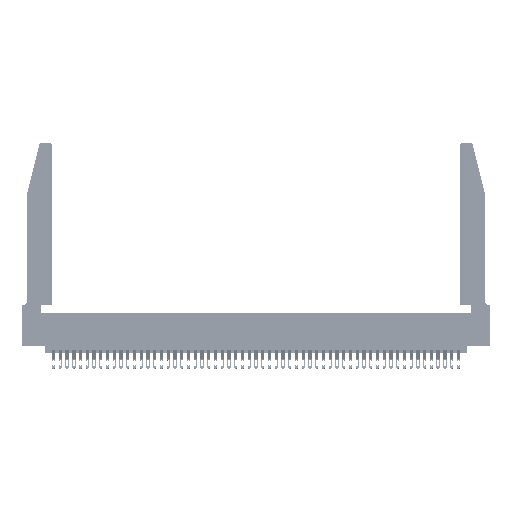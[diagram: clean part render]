
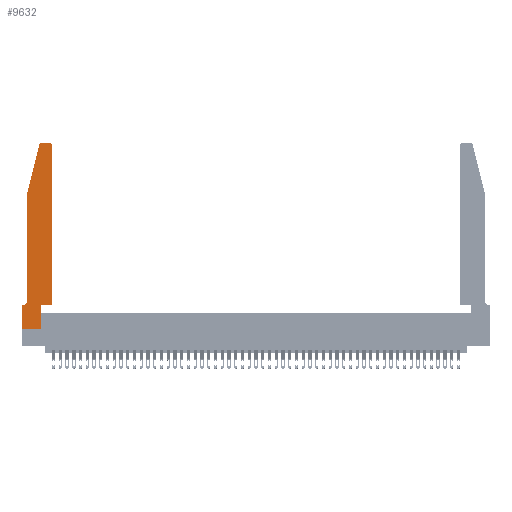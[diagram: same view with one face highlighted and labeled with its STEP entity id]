
A CAD part, top view. The second image highlights one B-rep face of the part: STEP entity #9632.
In plain terms, the highlighted planar face has unit normal (0, 0, 1).
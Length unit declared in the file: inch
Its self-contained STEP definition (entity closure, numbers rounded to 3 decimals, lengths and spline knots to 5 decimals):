
#800 = VERTEX_POINT ( 'NONE', #44283 ) ;
#1024 = ORIENTED_EDGE ( 'NONE', *, *, #45616, .T. ) ;
#1271 = VECTOR ( 'NONE', #14270, 39.37008 ) ;
#1954 = VERTEX_POINT ( 'NONE', #19782 ) ;
#2425 = EDGE_CURVE ( 'NONE', #1954, #8336, #3723, .T. ) ;
#2512 = LINE ( 'NONE', #45098, #1271 ) ;
#2571 = EDGE_CURVE ( 'NONE', #31086, #1954, #31881, .T. ) ;
#2613 = DIRECTION ( 'NONE',  ( 0., 0., 1. ) ) ;
#3529 = CIRCLE ( 'NONE', #30693, 0.07 ) ;
#3636 = EDGE_CURVE ( 'NONE', #43259, #8130, #29319, .T. ) ;
#3681 = VERTEX_POINT ( 'NONE', #5952 ) ;
#3723 = LINE ( 'NONE', #18517, #23317 ) ;
#5362 = DIRECTION ( 'NONE',  ( 0., 0., 1. ) ) ;
#5461 = AXIS2_PLACEMENT_3D ( 'NONE', #14263, #2613, #41509 ) ;
#5570 = PLANE ( 'NONE',  #5461 ) ;
#5894 = VECTOR ( 'NONE', #45492, 39.37008 ) ;
#5952 = CARTESIAN_POINT ( 'NONE',  ( 0.4205, 2.75, 0.37 ) ) ;
#6619 = AXIS2_PLACEMENT_3D ( 'NONE', #16443, #8090, #20015 ) ;
#6862 = CARTESIAN_POINT ( 'NONE',  ( 0.0055, 0.42, 0.37 ) ) ;
#7336 = EDGE_CURVE ( 'NONE', #8336, #18331, #37607, .T. ) ;
#8090 = DIRECTION ( 'NONE',  ( 0., 0., 1. ) ) ;
#8130 = VERTEX_POINT ( 'NONE', #14925 ) ;
#8336 = VERTEX_POINT ( 'NONE', #47598 ) ;
#8561 = LINE ( 'NONE', #13106, #26130 ) ;
#8973 = CARTESIAN_POINT ( 'NONE',  ( 0.0055, 0.35, 0.37 ) ) ;
#9632 = ADVANCED_FACE ( 'NONE', ( #42915 ), #5570, .T. ) ;
#10217 = CARTESIAN_POINT ( 'NONE',  ( 0.0755, 0.42, 0.37 ) ) ;
#10371 = LINE ( 'NONE', #47844, #37800 ) ;
#11352 = ORIENTED_EDGE ( 'NONE', *, *, #2425, .T. ) ;
#13106 = CARTESIAN_POINT ( 'NONE',  ( 0.0755, 2., 0.37 ) ) ;
#14122 = LINE ( 'NONE', #43935, #39158 ) ;
#14263 = CARTESIAN_POINT ( 'NONE',  ( 0., 0.35, 0.37 ) ) ;
#14270 = DIRECTION ( 'NONE',  ( 0., -1., 0. ) ) ;
#14535 = CARTESIAN_POINT ( 'NONE',  ( 0.284, 2.75, 0.37 ) ) ;
#14554 = DIRECTION ( 'NONE',  ( 0., 0., -1. ) ) ;
#14925 = CARTESIAN_POINT ( 'NONE',  ( 0.25487, 2.72718, 0.37 ) ) ;
#16443 = CARTESIAN_POINT ( 'NONE',  ( 0.4205, 2.72, 0.37 ) ) ;
#16849 = EDGE_LOOP ( 'NONE', ( #18432, #18050, #22694, #1024, #37319, #43086, #11352, #49983, #42268, #36477, #26808, #19203 ) ) ;
#18050 = ORIENTED_EDGE ( 'NONE', *, *, #3636, .T. ) ;
#18331 = VERTEX_POINT ( 'NONE', #22377 ) ;
#18432 = ORIENTED_EDGE ( 'NONE', *, *, #35262, .T. ) ;
#18517 = CARTESIAN_POINT ( 'NONE',  ( 0., 0., 0.37 ) ) ;
#19057 = CARTESIAN_POINT ( 'NONE',  ( 0.4505, 2.72, 0.37 ) ) ;
#19203 = ORIENTED_EDGE ( 'NONE', *, *, #32538, .T. ) ;
#19782 = CARTESIAN_POINT ( 'NONE',  ( 0., 0.35, 0.37 ) ) ;
#20015 = DIRECTION ( 'NONE',  ( 1., 0., 0. ) ) ;
#20072 = DIRECTION ( 'NONE',  ( 0., 1., 0. ) ) ;
#20753 = CARTESIAN_POINT ( 'NONE',  ( 0.284, 2.72, 0.37 ) ) ;
#20951 = DIRECTION ( 'NONE',  ( -1., 0., 0. ) ) ;
#21245 = DIRECTION ( 'NONE',  ( 1., 0., 0. ) ) ;
#22377 = CARTESIAN_POINT ( 'NONE',  ( 0.2865, 0., 0.37 ) ) ;
#22694 = ORIENTED_EDGE ( 'NONE', *, *, #35308, .T. ) ;
#22911 = DIRECTION ( 'NONE',  ( -1., 0., 0. ) ) ;
#23251 = VECTOR ( 'NONE', #26655, 39.37008 ) ;
#23317 = VECTOR ( 'NONE', #45058, 39.37008 ) ;
#23566 = CARTESIAN_POINT ( 'NONE',  ( 0.0755, 2., 0.37 ) ) ;
#24407 = EDGE_CURVE ( 'NONE', #38896, #43959, #36404, .T. ) ;
#26130 = VECTOR ( 'NONE', #48186, 39.37008 ) ;
#26391 = VECTOR ( 'NONE', #26518, 39.37008 ) ;
#26518 = DIRECTION ( 'NONE',  ( -1., 0., 0. ) ) ;
#26655 = DIRECTION ( 'NONE',  ( 1., 0., 0. ) ) ;
#26808 = ORIENTED_EDGE ( 'NONE', *, *, #24407, .T. ) ;
#26912 = LINE ( 'NONE', #37886, #23251 ) ;
#29319 = CIRCLE ( 'NONE', #31797, 0.03 ) ;
#30693 = AXIS2_PLACEMENT_3D ( 'NONE', #6862, #14554, #22911 ) ;
#31086 = VERTEX_POINT ( 'NONE', #8973 ) ;
#31797 = AXIS2_PLACEMENT_3D ( 'NONE', #20753, #5362, #21245 ) ;
#31881 = LINE ( 'NONE', #49802, #26391 ) ;
#32538 = EDGE_CURVE ( 'NONE', #43959, #3681, #38706, .T. ) ;
#33556 = CARTESIAN_POINT ( 'NONE',  ( 0.4505, 0.35, 0.37 ) ) ;
#35262 = EDGE_CURVE ( 'NONE', #3681, #43259, #10371, .T. ) ;
#35308 = EDGE_CURVE ( 'NONE', #8130, #36937, #8561, .T. ) ;
#36404 = LINE ( 'NONE', #44073, #41876 ) ;
#36477 = ORIENTED_EDGE ( 'NONE', *, *, #46283, .T. ) ;
#36937 = VERTEX_POINT ( 'NONE', #23566 ) ;
#37194 = EDGE_CURVE ( 'NONE', #18331, #800, #14122, .T. ) ;
#37319 = ORIENTED_EDGE ( 'NONE', *, *, #39734, .T. ) ;
#37607 = LINE ( 'NONE', #49068, #5894 ) ;
#37800 = VECTOR ( 'NONE', #20951, 39.37008 ) ;
#37886 = CARTESIAN_POINT ( 'NONE',  ( 0.4505, 0.35, 0.37 ) ) ;
#38706 = CIRCLE ( 'NONE', #6619, 0.03 ) ;
#38896 = VERTEX_POINT ( 'NONE', #33556 ) ;
#39158 = VECTOR ( 'NONE', #44936, 39.37008 ) ;
#39734 = EDGE_CURVE ( 'NONE', #45042, #31086, #3529, .T. ) ;
#41509 = DIRECTION ( 'NONE',  ( 1., 0., 0. ) ) ;
#41876 = VECTOR ( 'NONE', #20072, 39.37008 ) ;
#42268 = ORIENTED_EDGE ( 'NONE', *, *, #37194, .T. ) ;
#42915 = FACE_OUTER_BOUND ( 'NONE', #16849, .T. ) ;
#43086 = ORIENTED_EDGE ( 'NONE', *, *, #2571, .T. ) ;
#43259 = VERTEX_POINT ( 'NONE', #14535 ) ;
#43935 = CARTESIAN_POINT ( 'NONE',  ( 0.2865, 0.35, 0.37 ) ) ;
#43959 = VERTEX_POINT ( 'NONE', #19057 ) ;
#44073 = CARTESIAN_POINT ( 'NONE',  ( 0.4505, 0.35, 0.37 ) ) ;
#44283 = CARTESIAN_POINT ( 'NONE',  ( 0.2865, 0.35, 0.37 ) ) ;
#44936 = DIRECTION ( 'NONE',  ( 0., 1., 0. ) ) ;
#45042 = VERTEX_POINT ( 'NONE', #10217 ) ;
#45058 = DIRECTION ( 'NONE',  ( 0., -1., 0. ) ) ;
#45098 = CARTESIAN_POINT ( 'NONE',  ( 0.0755, 2., 0.37 ) ) ;
#45492 = DIRECTION ( 'NONE',  ( 1., 0., 0. ) ) ;
#45616 = EDGE_CURVE ( 'NONE', #36937, #45042, #2512, .T. ) ;
#46283 = EDGE_CURVE ( 'NONE', #800, #38896, #26912, .T. ) ;
#47598 = CARTESIAN_POINT ( 'NONE',  ( 0., 0., 0.37 ) ) ;
#47844 = CARTESIAN_POINT ( 'NONE',  ( 0.2605, 2.75, 0.37 ) ) ;
#48186 = DIRECTION ( 'NONE',  ( -0.239, -0.971, 0. ) ) ;
#49068 = CARTESIAN_POINT ( 'NONE',  ( 0., 0., 0.37 ) ) ;
#49802 = CARTESIAN_POINT ( 'NONE',  ( 0.0755, 0.35, 0.37 ) ) ;
#49983 = ORIENTED_EDGE ( 'NONE', *, *, #7336, .T. ) ;
